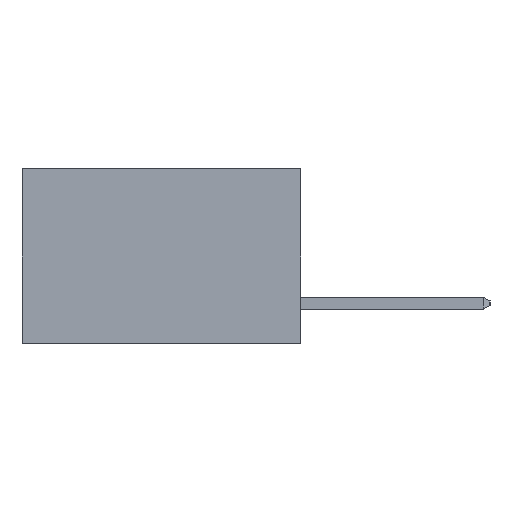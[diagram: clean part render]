
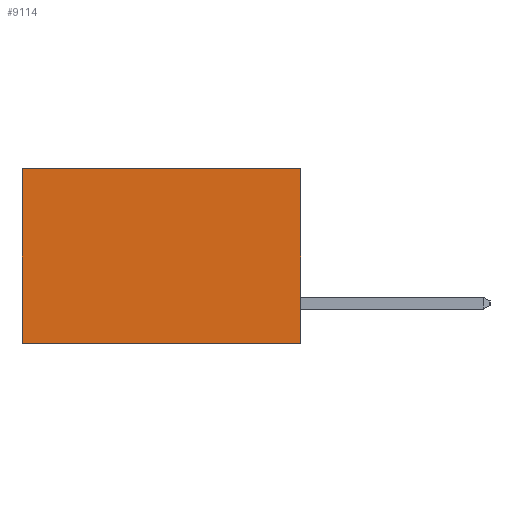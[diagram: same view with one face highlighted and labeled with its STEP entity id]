
A CAD part, left-side view. The second image highlights one B-rep face of the part: STEP entity #9114.
In plain terms, the highlighted planar face has unit normal (-1, 0, 0).
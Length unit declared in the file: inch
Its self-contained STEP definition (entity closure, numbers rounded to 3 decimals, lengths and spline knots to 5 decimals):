
#966 = CARTESIAN_POINT ( 'NONE',  ( 0.277, 0., 0. ) ) ;
#1242 = VERTEX_POINT ( 'NONE', #18152 ) ;
#1589 = VECTOR ( 'NONE', #29238, 39.37008 ) ;
#3013 = VERTEX_POINT ( 'NONE', #22240 ) ;
#3285 = DIRECTION ( 'NONE',  ( 0., 1., 0. ) ) ;
#5267 = EDGE_CURVE ( 'NONE', #27370, #15803, #22927, .T. ) ;
#5581 = DIRECTION ( 'NONE',  ( 0., 0., -1. ) ) ;
#7724 = VECTOR ( 'NONE', #18452, 39.37008 ) ;
#7901 = CARTESIAN_POINT ( 'NONE',  ( 0.277, 0., 0. ) ) ;
#8157 = EDGE_CURVE ( 'NONE', #27370, #1242, #20664, .T. ) ;
#8428 = ORIENTED_EDGE ( 'NONE', *, *, #24002, .T. ) ;
#8683 = ORIENTED_EDGE ( 'NONE', *, *, #8157, .F. ) ;
#9114 = ADVANCED_FACE ( 'NONE', ( #29031 ), #14771, .F. ) ;
#9181 = LINE ( 'NONE', #12844, #7724 ) ;
#10427 = LINE ( 'NONE', #12823, #22575 ) ;
#12823 = CARTESIAN_POINT ( 'NONE',  ( 0.277, 0.59, -0.37 ) ) ;
#12844 = CARTESIAN_POINT ( 'NONE',  ( 0.277, 0., -0.37 ) ) ;
#13074 = CARTESIAN_POINT ( 'NONE',  ( 0.277, 0.59, 0. ) ) ;
#13975 = EDGE_LOOP ( 'NONE', ( #8428, #17301, #8683, #23846 ) ) ;
#14771 = PLANE ( 'NONE',  #20676 ) ;
#15146 = DIRECTION ( 'NONE',  ( 0., 0., -1. ) ) ;
#15803 = VERTEX_POINT ( 'NONE', #13074 ) ;
#17063 = CARTESIAN_POINT ( 'NONE',  ( 0.277, 0., -0.37 ) ) ;
#17301 = ORIENTED_EDGE ( 'NONE', *, *, #26530, .F. ) ;
#17587 = VECTOR ( 'NONE', #3285, 39.37008 ) ;
#18152 = CARTESIAN_POINT ( 'NONE',  ( 0.277, 0., -0.37 ) ) ;
#18452 = DIRECTION ( 'NONE',  ( 0., 1., 0. ) ) ;
#19362 = DIRECTION ( 'NONE',  ( 1., 0., 0. ) ) ;
#20664 = LINE ( 'NONE', #27005, #1589 ) ;
#20676 = AXIS2_PLACEMENT_3D ( 'NONE', #17063, #19362, #5581 ) ;
#22240 = CARTESIAN_POINT ( 'NONE',  ( 0.277, 0.59, -0.37 ) ) ;
#22575 = VECTOR ( 'NONE', #15146, 39.37008 ) ;
#22927 = LINE ( 'NONE', #7901, #17587 ) ;
#23846 = ORIENTED_EDGE ( 'NONE', *, *, #5267, .T. ) ;
#24002 = EDGE_CURVE ( 'NONE', #15803, #3013, #10427, .T. ) ;
#26530 = EDGE_CURVE ( 'NONE', #1242, #3013, #9181, .T. ) ;
#27005 = CARTESIAN_POINT ( 'NONE',  ( 0.277, 0., -0.37 ) ) ;
#27370 = VERTEX_POINT ( 'NONE', #966 ) ;
#29031 = FACE_OUTER_BOUND ( 'NONE', #13975, .T. ) ;
#29238 = DIRECTION ( 'NONE',  ( 0., 0., -1. ) ) ;
